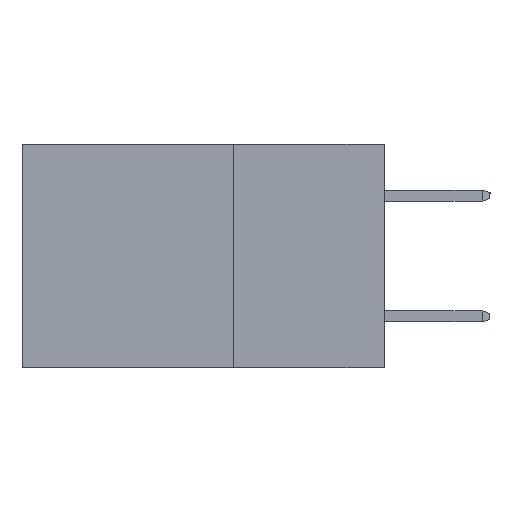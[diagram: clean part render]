
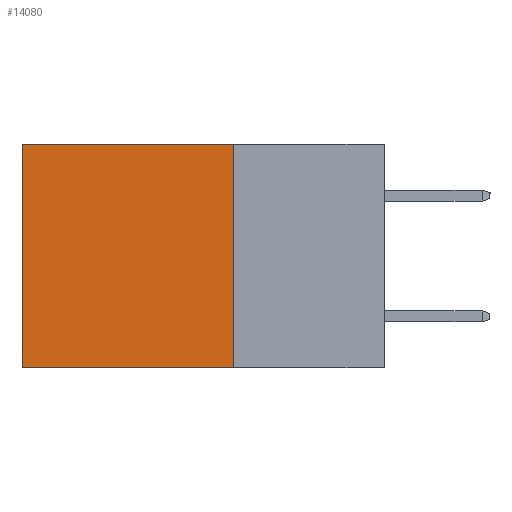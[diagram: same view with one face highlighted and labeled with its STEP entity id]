
A CAD part, left-side view. The second image highlights one B-rep face of the part: STEP entity #14080.
In plain terms, the highlighted planar face has unit normal (-1, 0, 0).
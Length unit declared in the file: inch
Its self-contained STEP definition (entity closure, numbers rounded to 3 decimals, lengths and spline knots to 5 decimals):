
#736 = DIRECTION ( 'NONE',  ( 0., 1., 0. ) ) ;
#767 = DIRECTION ( 'NONE',  ( 0., 0., -1. ) ) ;
#905 = CARTESIAN_POINT ( 'NONE',  ( 0.2615, 0.25, -0.37 ) ) ;
#1325 = VERTEX_POINT ( 'NONE', #1598 ) ;
#1598 = CARTESIAN_POINT ( 'NONE',  ( 0.2615, 0.25, -0.37 ) ) ;
#1750 = CARTESIAN_POINT ( 'NONE',  ( 0.2615, 0.25, 0. ) ) ;
#1799 = VERTEX_POINT ( 'NONE', #9045 ) ;
#2546 = LINE ( 'NONE', #905, #6217 ) ;
#2773 = CARTESIAN_POINT ( 'NONE',  ( 0.2615, 0.6, 0. ) ) ;
#2786 = VERTEX_POINT ( 'NONE', #2773 ) ;
#3213 = VECTOR ( 'NONE', #5327, 39.37008 ) ;
#3244 = EDGE_CURVE ( 'NONE', #2786, #14160, #8793, .T. ) ;
#3923 = ORIENTED_EDGE ( 'NONE', *, *, #9360, .T. ) ;
#4032 = EDGE_LOOP ( 'NONE', ( #7156, #9226, #10886, #3923 ) ) ;
#5059 = VECTOR ( 'NONE', #736, 39.37008 ) ;
#5327 = DIRECTION ( 'NONE',  ( 0., 0., -1. ) ) ;
#5809 = CARTESIAN_POINT ( 'NONE',  ( 0.2615, 0.6, -0.37 ) ) ;
#6217 = VECTOR ( 'NONE', #13988, 39.37008 ) ;
#6641 = LINE ( 'NONE', #12498, #9819 ) ;
#7156 = ORIENTED_EDGE ( 'NONE', *, *, #3244, .T. ) ;
#7569 = EDGE_CURVE ( 'NONE', #1799, #1325, #6641, .T. ) ;
#7991 = AXIS2_PLACEMENT_3D ( 'NONE', #12752, #13672, #767 ) ;
#8793 = LINE ( 'NONE', #13544, #3213 ) ;
#9045 = CARTESIAN_POINT ( 'NONE',  ( 0.2615, 0.25, 0. ) ) ;
#9226 = ORIENTED_EDGE ( 'NONE', *, *, #12849, .F. ) ;
#9360 = EDGE_CURVE ( 'NONE', #1799, #2786, #12719, .T. ) ;
#9819 = VECTOR ( 'NONE', #15068, 39.37008 ) ;
#10241 = FACE_OUTER_BOUND ( 'NONE', #4032, .T. ) ;
#10886 = ORIENTED_EDGE ( 'NONE', *, *, #7569, .F. ) ;
#11344 = PLANE ( 'NONE',  #7991 ) ;
#12498 = CARTESIAN_POINT ( 'NONE',  ( 0.2615, 0.25, -0.37 ) ) ;
#12719 = LINE ( 'NONE', #1750, #5059 ) ;
#12752 = CARTESIAN_POINT ( 'NONE',  ( 0.2615, 0.25, -0.37 ) ) ;
#12849 = EDGE_CURVE ( 'NONE', #1325, #14160, #2546, .T. ) ;
#13544 = CARTESIAN_POINT ( 'NONE',  ( 0.2615, 0.6, -0.37 ) ) ;
#13672 = DIRECTION ( 'NONE',  ( 1., 0., 0. ) ) ;
#13988 = DIRECTION ( 'NONE',  ( 0., 1., 0. ) ) ;
#14080 = ADVANCED_FACE ( 'NONE', ( #10241 ), #11344, .F. ) ;
#14160 = VERTEX_POINT ( 'NONE', #5809 ) ;
#15068 = DIRECTION ( 'NONE',  ( 0., 0., -1. ) ) ;
